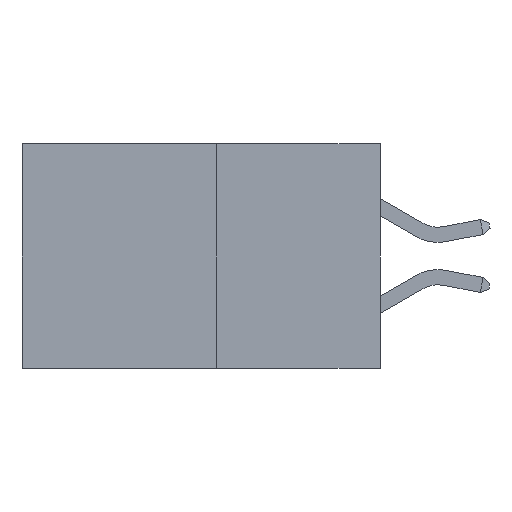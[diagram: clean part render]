
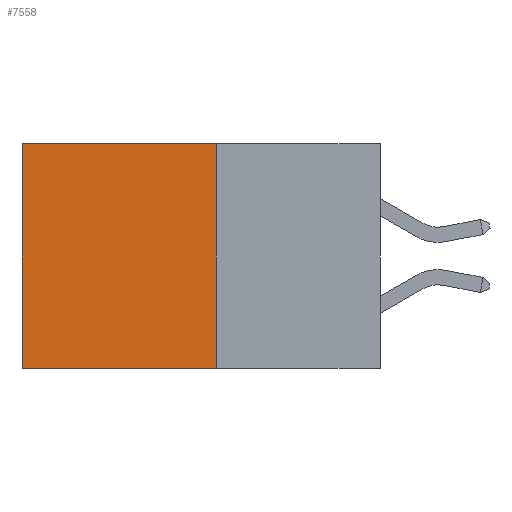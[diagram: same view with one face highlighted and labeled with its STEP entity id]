
A CAD part, left-side view. The second image highlights one B-rep face of the part: STEP entity #7558.
In plain terms, the highlighted planar face has unit normal (-1, 0, 0).
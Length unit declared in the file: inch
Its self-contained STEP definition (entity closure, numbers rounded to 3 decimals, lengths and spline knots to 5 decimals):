
#73 = ORIENTED_EDGE ( 'NONE', *, *, #21461, .T. ) ;
#171 = CARTESIAN_POINT ( 'NONE',  ( 0.277, 0.27, 0. ) ) ;
#1517 = VECTOR ( 'NONE', #2387, 39.37008 ) ;
#1633 = VERTEX_POINT ( 'NONE', #11984 ) ;
#2387 = DIRECTION ( 'NONE',  ( 0., 1., 0. ) ) ;
#4090 = CARTESIAN_POINT ( 'NONE',  ( 0.277, 0.59, -0.37 ) ) ;
#5317 = EDGE_LOOP ( 'NONE', ( #73, #11085, #17130, #12367 ) ) ;
#6449 = LINE ( 'NONE', #14729, #1517 ) ;
#6622 = VERTEX_POINT ( 'NONE', #4090 ) ;
#7040 = CARTESIAN_POINT ( 'NONE',  ( 0.277, 0.27, -0.37 ) ) ;
#7558 = ADVANCED_FACE ( 'NONE', ( #24747 ), #16077, .F. ) ;
#7970 = DIRECTION ( 'NONE',  ( 0., 0., -1. ) ) ;
#7979 = LINE ( 'NONE', #8424, #23357 ) ;
#8424 = CARTESIAN_POINT ( 'NONE',  ( 0.277, 0.59, -0.37 ) ) ;
#9069 = DIRECTION ( 'NONE',  ( 0., 0., -1. ) ) ;
#9206 = EDGE_CURVE ( 'NONE', #15654, #1633, #15911, .T. ) ;
#9251 = VECTOR ( 'NONE', #9613, 39.37008 ) ;
#9613 = DIRECTION ( 'NONE',  ( 0., 1., 0. ) ) ;
#9633 = AXIS2_PLACEMENT_3D ( 'NONE', #18066, #20049, #7970 ) ;
#9898 = LINE ( 'NONE', #19631, #9251 ) ;
#10489 = DIRECTION ( 'NONE',  ( 0., 0., -1. ) ) ;
#11085 = ORIENTED_EDGE ( 'NONE', *, *, #20155, .F. ) ;
#11984 = CARTESIAN_POINT ( 'NONE',  ( 0.277, 0.27, -0.37 ) ) ;
#12367 = ORIENTED_EDGE ( 'NONE', *, *, #22478, .T. ) ;
#14729 = CARTESIAN_POINT ( 'NONE',  ( 0.277, 0.27, -0.37 ) ) ;
#15654 = VERTEX_POINT ( 'NONE', #171 ) ;
#15702 = VERTEX_POINT ( 'NONE', #18694 ) ;
#15911 = LINE ( 'NONE', #7040, #25802 ) ;
#16077 = PLANE ( 'NONE',  #9633 ) ;
#17130 = ORIENTED_EDGE ( 'NONE', *, *, #9206, .F. ) ;
#18066 = CARTESIAN_POINT ( 'NONE',  ( 0.277, 0.27, -0.37 ) ) ;
#18694 = CARTESIAN_POINT ( 'NONE',  ( 0.277, 0.59, 0. ) ) ;
#19631 = CARTESIAN_POINT ( 'NONE',  ( 0.277, 0.27, 0. ) ) ;
#20049 = DIRECTION ( 'NONE',  ( 1., 0., 0. ) ) ;
#20155 = EDGE_CURVE ( 'NONE', #1633, #6622, #6449, .T. ) ;
#21461 = EDGE_CURVE ( 'NONE', #15702, #6622, #7979, .T. ) ;
#22478 = EDGE_CURVE ( 'NONE', #15654, #15702, #9898, .T. ) ;
#23357 = VECTOR ( 'NONE', #10489, 39.37008 ) ;
#24747 = FACE_OUTER_BOUND ( 'NONE', #5317, .T. ) ;
#25802 = VECTOR ( 'NONE', #9069, 39.37008 ) ;
